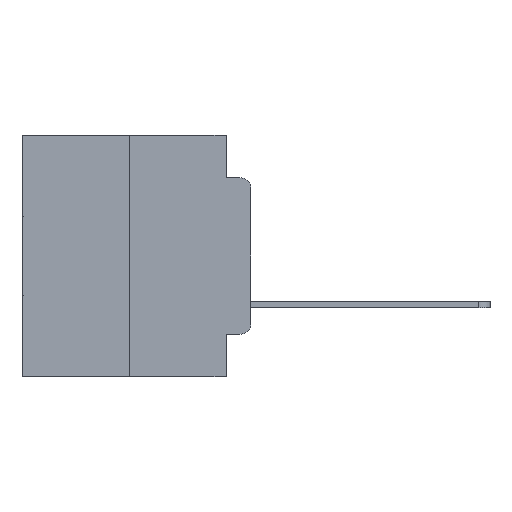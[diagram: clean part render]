
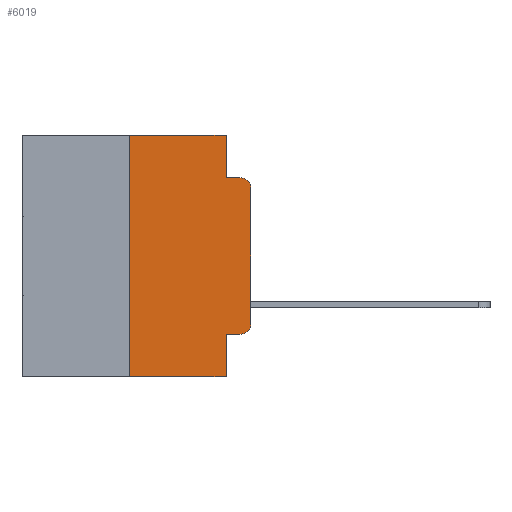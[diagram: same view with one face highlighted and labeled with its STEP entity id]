
A CAD part, left-side view. The second image highlights one B-rep face of the part: STEP entity #6019.
In plain terms, the highlighted planar face has unit normal (-1, 0, 0).
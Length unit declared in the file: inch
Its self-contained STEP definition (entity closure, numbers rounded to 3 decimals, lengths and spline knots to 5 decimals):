
#142 = CARTESIAN_POINT ( 'NONE',  ( 0., 0.02, -0.1085 ) ) ;
#572 = DIRECTION ( 'NONE',  ( 0., 0., 1. ) ) ;
#977 = LINE ( 'NONE', #17618, #9354 ) ;
#1256 = EDGE_CURVE ( 'NONE', #17661, #26865, #15144, .T. ) ;
#1318 = VERTEX_POINT ( 'NONE', #12758 ) ;
#1909 = CARTESIAN_POINT ( 'NONE',  ( 0., 0.051, -0.4115 ) ) ;
#3020 = CARTESIAN_POINT ( 'NONE',  ( 0., 0., 0. ) ) ;
#3725 = VECTOR ( 'NONE', #15291, 39.37008 ) ;
#3988 = VECTOR ( 'NONE', #4481, 39.37008 ) ;
#4068 = LINE ( 'NONE', #26189, #15789 ) ;
#4231 = VERTEX_POINT ( 'NONE', #22539 ) ;
#4308 = CARTESIAN_POINT ( 'NONE',  ( 0., 0.051, 0. ) ) ;
#4481 = DIRECTION ( 'NONE',  ( 0., 0., -1. ) ) ;
#5411 = CARTESIAN_POINT ( 'NONE',  ( 0., 0.051, 0. ) ) ;
#5502 = DIRECTION ( 'NONE',  ( 0., 0., -1. ) ) ;
#5974 = EDGE_CURVE ( 'NONE', #11691, #4231, #26592, .T. ) ;
#6019 = ADVANCED_FACE ( 'NONE', ( #12389 ), #24607, .F. ) ;
#6295 = LINE ( 'NONE', #18336, #22783 ) ;
#6461 = CARTESIAN_POINT ( 'NONE',  ( 0., 0.25, -0.5 ) ) ;
#7295 = AXIS2_PLACEMENT_3D ( 'NONE', #142, #8763, #15156 ) ;
#7548 = EDGE_CURVE ( 'NONE', #17661, #17870, #15721, .T. ) ;
#7649 = DIRECTION ( 'NONE',  ( 0., -1., 0. ) ) ;
#8103 = ORIENTED_EDGE ( 'NONE', *, *, #21743, .T. ) ;
#8763 = DIRECTION ( 'NONE',  ( -1., 0., 0. ) ) ;
#8971 = CARTESIAN_POINT ( 'NONE',  ( 0., 0.25, 0. ) ) ;
#9153 = DIRECTION ( 'NONE',  ( 0., -1., 0. ) ) ;
#9354 = VECTOR ( 'NONE', #9153, 39.37008 ) ;
#9721 = ORIENTED_EDGE ( 'NONE', *, *, #22250, .T. ) ;
#10634 = EDGE_CURVE ( 'NONE', #26865, #11691, #4068, .T. ) ;
#11079 = ORIENTED_EDGE ( 'NONE', *, *, #22788, .F. ) ;
#11411 = VECTOR ( 'NONE', #572, 39.37008 ) ;
#11552 = VERTEX_POINT ( 'NONE', #13018 ) ;
#11644 = EDGE_CURVE ( 'NONE', #25697, #13285, #977, .T. ) ;
#11688 = CARTESIAN_POINT ( 'NONE',  ( 0., 0.051, -0.5 ) ) ;
#11691 = VERTEX_POINT ( 'NONE', #15828 ) ;
#11910 = VERTEX_POINT ( 'NONE', #26745 ) ;
#12305 = CARTESIAN_POINT ( 'NONE',  ( 0., 0.02, -0.4115 ) ) ;
#12389 = FACE_OUTER_BOUND ( 'NONE', #12468, .T. ) ;
#12468 = EDGE_LOOP ( 'NONE', ( #8103, #14610, #27933, #15947, #25888, #18987, #24457, #11079, #16160, #9721 ) ) ;
#12758 = CARTESIAN_POINT ( 'NONE',  ( 0., 0., -0.1085 ) ) ;
#13018 = CARTESIAN_POINT ( 'NONE',  ( 0., 0.02, -0.0885 ) ) ;
#13271 = CARTESIAN_POINT ( 'NONE',  ( 0., 0.473, -0.5 ) ) ;
#13285 = VERTEX_POINT ( 'NONE', #12305 ) ;
#13454 = DIRECTION ( 'NONE',  ( 0., -1., 0. ) ) ;
#14610 = ORIENTED_EDGE ( 'NONE', *, *, #25358, .T. ) ;
#15136 = AXIS2_PLACEMENT_3D ( 'NONE', #23873, #15293, #26263 ) ;
#15144 = LINE ( 'NONE', #17437, #3725 ) ;
#15156 = DIRECTION ( 'NONE',  ( 0., 0., -1. ) ) ;
#15291 = DIRECTION ( 'NONE',  ( 0., 0., 1. ) ) ;
#15293 = DIRECTION ( 'NONE',  ( -1., 0., 0. ) ) ;
#15721 = LINE ( 'NONE', #13271, #25190 ) ;
#15789 = VECTOR ( 'NONE', #22093, 39.37008 ) ;
#15828 = CARTESIAN_POINT ( 'NONE',  ( 0., 0.051, 0. ) ) ;
#15947 = ORIENTED_EDGE ( 'NONE', *, *, #5974, .F. ) ;
#16160 = ORIENTED_EDGE ( 'NONE', *, *, #11644, .T. ) ;
#16428 = VECTOR ( 'NONE', #22355, 39.37008 ) ;
#17437 = CARTESIAN_POINT ( 'NONE',  ( 0., 0.25, 0. ) ) ;
#17618 = CARTESIAN_POINT ( 'NONE',  ( 0., 0.051, -0.4115 ) ) ;
#17661 = VERTEX_POINT ( 'NONE', #6461 ) ;
#17870 = VERTEX_POINT ( 'NONE', #11688 ) ;
#18175 = DIRECTION ( 'NONE',  ( 1., 0., 0. ) ) ;
#18336 = CARTESIAN_POINT ( 'NONE',  ( 0., 0.051, -0.0885 ) ) ;
#18365 = CARTESIAN_POINT ( 'NONE',  ( 0., 0.473, 0. ) ) ;
#18987 = ORIENTED_EDGE ( 'NONE', *, *, #1256, .F. ) ;
#19342 = AXIS2_PLACEMENT_3D ( 'NONE', #18365, #18175, #5502 ) ;
#20463 = CIRCLE ( 'NONE', #15136, 0.02 ) ;
#21743 = EDGE_CURVE ( 'NONE', #11910, #1318, #26294, .T. ) ;
#22093 = DIRECTION ( 'NONE',  ( 0., -1., 0. ) ) ;
#22250 = EDGE_CURVE ( 'NONE', #13285, #11910, #20463, .T. ) ;
#22355 = DIRECTION ( 'NONE',  ( 0., 0., -1. ) ) ;
#22539 = CARTESIAN_POINT ( 'NONE',  ( 0., 0.051, -0.0885 ) ) ;
#22783 = VECTOR ( 'NONE', #7649, 39.37008 ) ;
#22788 = EDGE_CURVE ( 'NONE', #25697, #17870, #23172, .T. ) ;
#23172 = LINE ( 'NONE', #4308, #3988 ) ;
#23873 = CARTESIAN_POINT ( 'NONE',  ( 0., 0.02, -0.3915 ) ) ;
#24457 = ORIENTED_EDGE ( 'NONE', *, *, #7548, .T. ) ;
#24607 = PLANE ( 'NONE',  #19342 ) ;
#25190 = VECTOR ( 'NONE', #13454, 39.37008 ) ;
#25248 = CIRCLE ( 'NONE', #7295, 0.02 ) ;
#25358 = EDGE_CURVE ( 'NONE', #1318, #11552, #25248, .T. ) ;
#25697 = VERTEX_POINT ( 'NONE', #1909 ) ;
#25888 = ORIENTED_EDGE ( 'NONE', *, *, #10634, .F. ) ;
#26189 = CARTESIAN_POINT ( 'NONE',  ( 0., 0.473, 0. ) ) ;
#26263 = DIRECTION ( 'NONE',  ( 0., 0., -1. ) ) ;
#26294 = LINE ( 'NONE', #3020, #11411 ) ;
#26592 = LINE ( 'NONE', #5411, #16428 ) ;
#26745 = CARTESIAN_POINT ( 'NONE',  ( 0., 0., -0.3915 ) ) ;
#26865 = VERTEX_POINT ( 'NONE', #8971 ) ;
#27678 = EDGE_CURVE ( 'NONE', #4231, #11552, #6295, .T. ) ;
#27933 = ORIENTED_EDGE ( 'NONE', *, *, #27678, .F. ) ;
